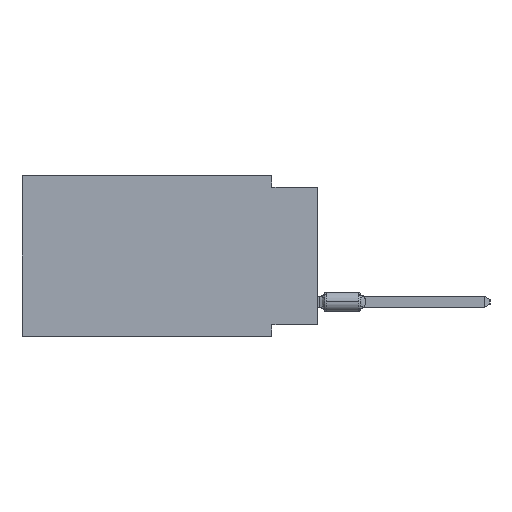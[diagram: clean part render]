
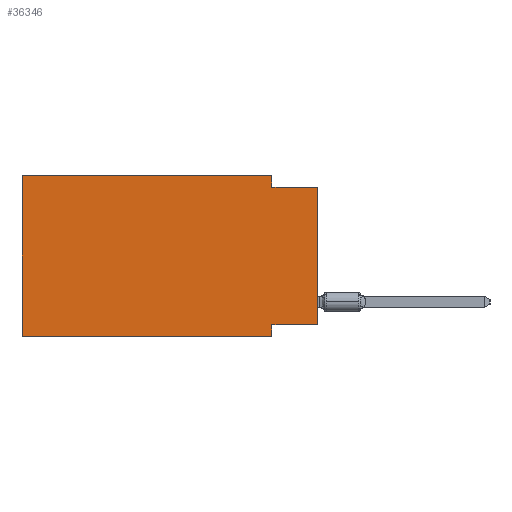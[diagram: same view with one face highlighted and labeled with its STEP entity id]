
A CAD part, left-side view. The second image highlights one B-rep face of the part: STEP entity #36346.
In plain terms, the highlighted planar face has unit normal (-1, 0, 0).
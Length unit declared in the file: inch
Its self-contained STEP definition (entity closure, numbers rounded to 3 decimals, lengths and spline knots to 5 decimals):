
#3854 = DIRECTION ( 'NONE',  ( 0., -1., 0. ) ) ;
#3972 = CARTESIAN_POINT ( 'NONE',  ( 0., 0., 0. ) ) ;
#4822 = FACE_OUTER_BOUND ( 'NONE', #47225, .T. ) ;
#5056 = CARTESIAN_POINT ( 'NONE',  ( 0., 0.645, 0. ) ) ;
#5222 = CARTESIAN_POINT ( 'NONE',  ( 0., 0., -0.325 ) ) ;
#5990 = ORIENTED_EDGE ( 'NONE', *, *, #15243, .F. ) ;
#6383 = CARTESIAN_POINT ( 'NONE',  ( 0., 0.645, 0. ) ) ;
#6641 = VERTEX_POINT ( 'NONE', #37076 ) ;
#6867 = CARTESIAN_POINT ( 'NONE',  ( 0., 0., -0.025 ) ) ;
#9696 = LINE ( 'NONE', #30337, #28622 ) ;
#10146 = DIRECTION ( 'NONE',  ( 0., 1., 0. ) ) ;
#10950 = VERTEX_POINT ( 'NONE', #60821 ) ;
#10954 = DIRECTION ( 'NONE',  ( 0., -1., 0. ) ) ;
#12627 = DIRECTION ( 'NONE',  ( 0., 0., -1. ) ) ;
#13248 = VECTOR ( 'NONE', #40143, 39.37008 ) ;
#14544 = VECTOR ( 'NONE', #34113, 39.37008 ) ;
#15243 = EDGE_CURVE ( 'NONE', #67955, #6641, #44103, .T. ) ;
#17065 = VECTOR ( 'NONE', #10954, 39.37008 ) ;
#17555 = ORIENTED_EDGE ( 'NONE', *, *, #25286, .F. ) ;
#18097 = EDGE_CURVE ( 'NONE', #65919, #66268, #57164, .T. ) ;
#21446 = EDGE_CURVE ( 'NONE', #51558, #10950, #56585, .T. ) ;
#22286 = CARTESIAN_POINT ( 'NONE',  ( 0., 0.1, -0.325 ) ) ;
#22586 = CARTESIAN_POINT ( 'NONE',  ( 0., 0., -0.025 ) ) ;
#25286 = EDGE_CURVE ( 'NONE', #10950, #66268, #49539, .T. ) ;
#25327 = DIRECTION ( 'NONE',  ( 0., 0., 1. ) ) ;
#26694 = LINE ( 'NONE', #6383, #17065 ) ;
#27202 = DIRECTION ( 'NONE',  ( 1., 0., 0. ) ) ;
#27524 = EDGE_CURVE ( 'NONE', #65919, #67955, #41616, .T. ) ;
#28622 = VECTOR ( 'NONE', #67751, 39.37008 ) ;
#29298 = VERTEX_POINT ( 'NONE', #44596 ) ;
#29565 = CARTESIAN_POINT ( 'NONE',  ( 0., 0.1, 0. ) ) ;
#30337 = CARTESIAN_POINT ( 'NONE',  ( 0., 0.645, 0. ) ) ;
#30936 = EDGE_CURVE ( 'NONE', #52878, #51558, #26694, .T. ) ;
#31730 = ORIENTED_EDGE ( 'NONE', *, *, #52448, .T. ) ;
#31828 = VECTOR ( 'NONE', #25327, 39.37008 ) ;
#33995 = VECTOR ( 'NONE', #12627, 39.37008 ) ;
#34113 = DIRECTION ( 'NONE',  ( 0., -1., 0. ) ) ;
#36346 = ADVANCED_FACE ( 'NONE', ( #4822 ), #43301, .F. ) ;
#37066 = VECTOR ( 'NONE', #10146, 39.37008 ) ;
#37076 = CARTESIAN_POINT ( 'NONE',  ( 0., 0.1, -0.35 ) ) ;
#40143 = DIRECTION ( 'NONE',  ( 0., 0., -1. ) ) ;
#40491 = CARTESIAN_POINT ( 'NONE',  ( 0., 0.1, 0. ) ) ;
#40590 = LINE ( 'NONE', #52810, #42705 ) ;
#41330 = ORIENTED_EDGE ( 'NONE', *, *, #27524, .F. ) ;
#41616 = LINE ( 'NONE', #5222, #37066 ) ;
#42705 = VECTOR ( 'NONE', #3854, 39.37008 ) ;
#43266 = AXIS2_PLACEMENT_3D ( 'NONE', #53100, #27202, #53437 ) ;
#43301 = PLANE ( 'NONE',  #43266 ) ;
#44103 = LINE ( 'NONE', #55285, #33995 ) ;
#44596 = CARTESIAN_POINT ( 'NONE',  ( 0., 0.645, -0.35 ) ) ;
#47225 = EDGE_LOOP ( 'NONE', ( #55143, #17555, #61915, #68124, #61318, #31730, #5990, #41330 ) ) ;
#49539 = LINE ( 'NONE', #6867, #14544 ) ;
#51558 = VERTEX_POINT ( 'NONE', #29565 ) ;
#52324 = CARTESIAN_POINT ( 'NONE',  ( 0., 0., -0.325 ) ) ;
#52448 = EDGE_CURVE ( 'NONE', #29298, #6641, #40590, .T. ) ;
#52810 = CARTESIAN_POINT ( 'NONE',  ( 0., 0.645, -0.35 ) ) ;
#52878 = VERTEX_POINT ( 'NONE', #5056 ) ;
#53100 = CARTESIAN_POINT ( 'NONE',  ( 0., 0.645, 0. ) ) ;
#53437 = DIRECTION ( 'NONE',  ( 0., 0., -1. ) ) ;
#55143 = ORIENTED_EDGE ( 'NONE', *, *, #18097, .T. ) ;
#55285 = CARTESIAN_POINT ( 'NONE',  ( 0., 0.1, -0.35 ) ) ;
#56585 = LINE ( 'NONE', #40491, #13248 ) ;
#57164 = LINE ( 'NONE', #3972, #31828 ) ;
#60821 = CARTESIAN_POINT ( 'NONE',  ( 0., 0.1, -0.025 ) ) ;
#61318 = ORIENTED_EDGE ( 'NONE', *, *, #67798, .F. ) ;
#61915 = ORIENTED_EDGE ( 'NONE', *, *, #21446, .F. ) ;
#65919 = VERTEX_POINT ( 'NONE', #52324 ) ;
#66268 = VERTEX_POINT ( 'NONE', #22586 ) ;
#67751 = DIRECTION ( 'NONE',  ( 0., 0., 1. ) ) ;
#67798 = EDGE_CURVE ( 'NONE', #29298, #52878, #9696, .T. ) ;
#67955 = VERTEX_POINT ( 'NONE', #22286 ) ;
#68124 = ORIENTED_EDGE ( 'NONE', *, *, #30936, .F. ) ;
